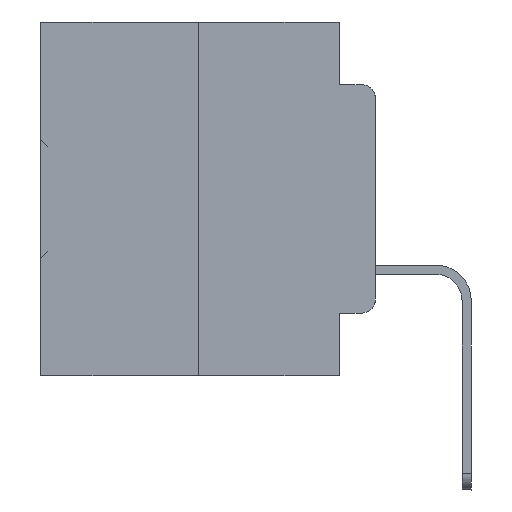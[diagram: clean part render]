
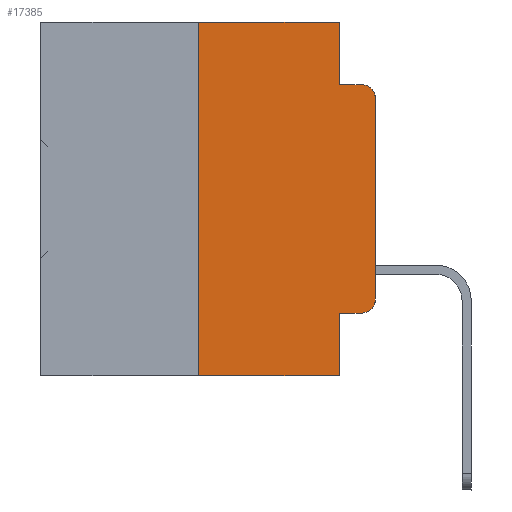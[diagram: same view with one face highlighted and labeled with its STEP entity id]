
A CAD part, left-side view. The second image highlights one B-rep face of the part: STEP entity #17385.
In plain terms, the highlighted planar face has unit normal (-1, 0, 0).
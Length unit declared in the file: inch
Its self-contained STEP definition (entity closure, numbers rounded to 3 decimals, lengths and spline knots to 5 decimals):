
#253 = EDGE_CURVE ( 'NONE', #3105, #2087, #5118, .T. ) ;
#779 = EDGE_CURVE ( 'NONE', #6967, #20923, #25473, .T. ) ;
#1698 = VECTOR ( 'NONE', #4354, 39.37008 ) ;
#1738 = FACE_OUTER_BOUND ( 'NONE', #24714, .T. ) ;
#1805 = AXIS2_PLACEMENT_3D ( 'NONE', #31427, #31304, #31673 ) ;
#2087 = VERTEX_POINT ( 'NONE', #2591 ) ;
#2120 = DIRECTION ( 'NONE',  ( 0., 0., -1. ) ) ;
#2338 = CARTESIAN_POINT ( 'NONE',  ( 0., 0.051, -0.4115 ) ) ;
#2591 = CARTESIAN_POINT ( 'NONE',  ( 0., 0.051, -0.0885 ) ) ;
#2632 = LINE ( 'NONE', #23409, #5853 ) ;
#2800 = ORIENTED_EDGE ( 'NONE', *, *, #253, .F. ) ;
#3099 = AXIS2_PLACEMENT_3D ( 'NONE', #8784, #3110, #20329 ) ;
#3105 = VERTEX_POINT ( 'NONE', #9837 ) ;
#3110 = DIRECTION ( 'NONE',  ( -1., 0., 0. ) ) ;
#3297 = VECTOR ( 'NONE', #20672, 39.37008 ) ;
#3324 = VERTEX_POINT ( 'NONE', #5275 ) ;
#4354 = DIRECTION ( 'NONE',  ( 0., -1., 0. ) ) ;
#5118 = LINE ( 'NONE', #9279, #3297 ) ;
#5275 = CARTESIAN_POINT ( 'NONE',  ( 0., 0.02, -0.4115 ) ) ;
#5810 = LINE ( 'NONE', #25294, #12560 ) ;
#5853 = VECTOR ( 'NONE', #32920, 39.37008 ) ;
#6967 = VERTEX_POINT ( 'NONE', #21155 ) ;
#7962 = EDGE_CURVE ( 'NONE', #9109, #28802, #21038, .T. ) ;
#8078 = EDGE_CURVE ( 'NONE', #3324, #9685, #11501, .T. ) ;
#8784 = CARTESIAN_POINT ( 'NONE',  ( 0., 0.02, -0.1085 ) ) ;
#9109 = VERTEX_POINT ( 'NONE', #33891 ) ;
#9279 = CARTESIAN_POINT ( 'NONE',  ( 0., 0.051, 0. ) ) ;
#9685 = VERTEX_POINT ( 'NONE', #16825 ) ;
#9837 = CARTESIAN_POINT ( 'NONE',  ( 0., 0.051, 0. ) ) ;
#10587 = CARTESIAN_POINT ( 'NONE',  ( 0., 0.051, -0.5 ) ) ;
#11001 = EDGE_CURVE ( 'NONE', #2087, #28802, #12341, .T. ) ;
#11345 = VECTOR ( 'NONE', #28533, 39.37008 ) ;
#11440 = CARTESIAN_POINT ( 'NONE',  ( 0., 0.02, -0.3915 ) ) ;
#11501 = CIRCLE ( 'NONE', #24474, 0.02 ) ;
#12341 = LINE ( 'NONE', #22843, #31882 ) ;
#12560 = VECTOR ( 'NONE', #2120, 39.37008 ) ;
#13233 = CARTESIAN_POINT ( 'NONE',  ( 0., 0.473, -0.5 ) ) ;
#13374 = EDGE_CURVE ( 'NONE', #29580, #3105, #2632, .T. ) ;
#13660 = EDGE_CURVE ( 'NONE', #23213, #20923, #5810, .T. ) ;
#14032 = EDGE_CURVE ( 'NONE', #23213, #3324, #35267, .T. ) ;
#15239 = CARTESIAN_POINT ( 'NONE',  ( 0., 0., 0. ) ) ;
#16825 = CARTESIAN_POINT ( 'NONE',  ( 0., 0., -0.3915 ) ) ;
#16858 = DIRECTION ( 'NONE',  ( 0., -1., 0. ) ) ;
#17385 = ADVANCED_FACE ( 'NONE', ( #1738 ), #22518, .F. ) ;
#18096 = CARTESIAN_POINT ( 'NONE',  ( 0., 0.02, -0.0885 ) ) ;
#20329 = DIRECTION ( 'NONE',  ( 0., 0., -1. ) ) ;
#20449 = DIRECTION ( 'NONE',  ( 0., 0., -1. ) ) ;
#20672 = DIRECTION ( 'NONE',  ( 0., 0., -1. ) ) ;
#20923 = VERTEX_POINT ( 'NONE', #10587 ) ;
#20968 = DIRECTION ( 'NONE',  ( 0., 0., 1. ) ) ;
#21038 = CIRCLE ( 'NONE', #3099, 0.02 ) ;
#21155 = CARTESIAN_POINT ( 'NONE',  ( 0., 0.25, -0.5 ) ) ;
#21862 = LINE ( 'NONE', #15239, #30028 ) ;
#22124 = ORIENTED_EDGE ( 'NONE', *, *, #11001, .F. ) ;
#22518 = PLANE ( 'NONE',  #1805 ) ;
#22843 = CARTESIAN_POINT ( 'NONE',  ( 0., 0.051, -0.0885 ) ) ;
#23130 = ORIENTED_EDGE ( 'NONE', *, *, #13374, .F. ) ;
#23213 = VERTEX_POINT ( 'NONE', #2338 ) ;
#23409 = CARTESIAN_POINT ( 'NONE',  ( 0., 0.473, 0. ) ) ;
#24474 = AXIS2_PLACEMENT_3D ( 'NONE', #11440, #29329, #20449 ) ;
#24714 = EDGE_LOOP ( 'NONE', ( #30907, #37243, #22124, #2800, #23130, #28517, #34172, #26241, #24850, #26595 ) ) ;
#24850 = ORIENTED_EDGE ( 'NONE', *, *, #14032, .T. ) ;
#25294 = CARTESIAN_POINT ( 'NONE',  ( 0., 0.051, 0. ) ) ;
#25473 = LINE ( 'NONE', #13233, #36789 ) ;
#26241 = ORIENTED_EDGE ( 'NONE', *, *, #13660, .F. ) ;
#26595 = ORIENTED_EDGE ( 'NONE', *, *, #8078, .T. ) ;
#28517 = ORIENTED_EDGE ( 'NONE', *, *, #36080, .F. ) ;
#28533 = DIRECTION ( 'NONE',  ( 0., 0., 1. ) ) ;
#28802 = VERTEX_POINT ( 'NONE', #18096 ) ;
#29329 = DIRECTION ( 'NONE',  ( -1., 0., 0. ) ) ;
#29528 = LINE ( 'NONE', #34238, #11345 ) ;
#29580 = VERTEX_POINT ( 'NONE', #31553 ) ;
#30028 = VECTOR ( 'NONE', #20968, 39.37008 ) ;
#30351 = CARTESIAN_POINT ( 'NONE',  ( 0., 0.051, -0.4115 ) ) ;
#30659 = DIRECTION ( 'NONE',  ( 0., -1., 0. ) ) ;
#30907 = ORIENTED_EDGE ( 'NONE', *, *, #35136, .T. ) ;
#31304 = DIRECTION ( 'NONE',  ( 1., 0., 0. ) ) ;
#31427 = CARTESIAN_POINT ( 'NONE',  ( 0., 0.473, 0. ) ) ;
#31553 = CARTESIAN_POINT ( 'NONE',  ( 0., 0.25, 0. ) ) ;
#31673 = DIRECTION ( 'NONE',  ( 0., 0., -1. ) ) ;
#31882 = VECTOR ( 'NONE', #16858, 39.37008 ) ;
#32920 = DIRECTION ( 'NONE',  ( 0., -1., 0. ) ) ;
#33891 = CARTESIAN_POINT ( 'NONE',  ( 0., 0., -0.1085 ) ) ;
#34172 = ORIENTED_EDGE ( 'NONE', *, *, #779, .T. ) ;
#34238 = CARTESIAN_POINT ( 'NONE',  ( 0., 0.25, 0. ) ) ;
#35136 = EDGE_CURVE ( 'NONE', #9685, #9109, #21862, .T. ) ;
#35267 = LINE ( 'NONE', #30351, #1698 ) ;
#36080 = EDGE_CURVE ( 'NONE', #6967, #29580, #29528, .T. ) ;
#36789 = VECTOR ( 'NONE', #30659, 39.37008 ) ;
#37243 = ORIENTED_EDGE ( 'NONE', *, *, #7962, .T. ) ;
